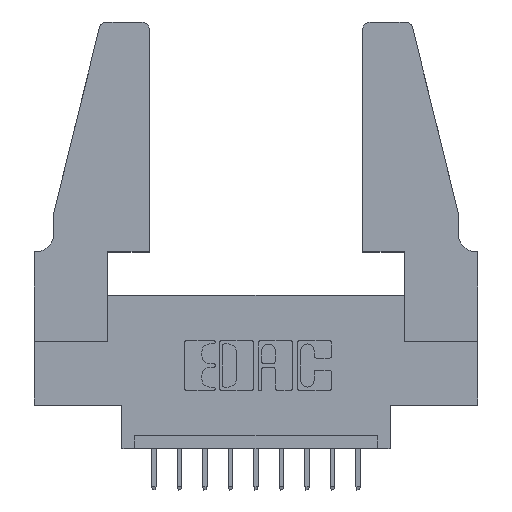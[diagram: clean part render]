
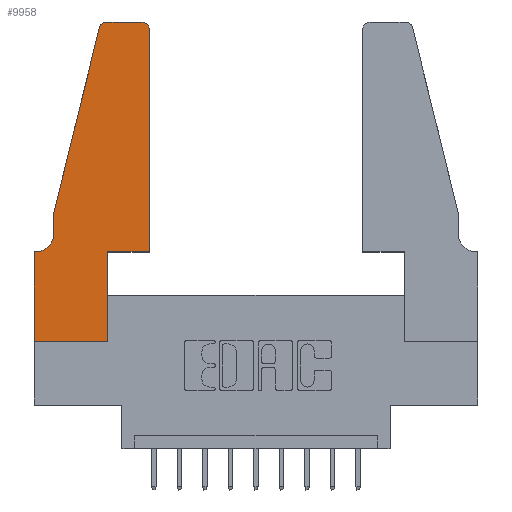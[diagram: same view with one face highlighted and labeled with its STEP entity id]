
A CAD part, top view. The second image highlights one B-rep face of the part: STEP entity #9958.
In plain terms, the highlighted planar face has unit normal (0, 0, 1).
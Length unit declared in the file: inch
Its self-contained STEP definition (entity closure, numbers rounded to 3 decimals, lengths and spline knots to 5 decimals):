
#3 = ORIENTED_EDGE ( 'NONE', *, *, #6358, .T. ) ;
#134 = CARTESIAN_POINT ( 'NONE',  ( 0.0755, 0.35, 0.37 ) ) ;
#165 = LINE ( 'NONE', #5622, #8355 ) ;
#537 = VERTEX_POINT ( 'NONE', #12414 ) ;
#626 = CARTESIAN_POINT ( 'NONE',  ( 0.0055, 0.42, 0.37 ) ) ;
#753 = CARTESIAN_POINT ( 'NONE',  ( 0.2865, 0.35, 0.37 ) ) ;
#811 = AXIS2_PLACEMENT_3D ( 'NONE', #626, #10054, #12198 ) ;
#1028 = VECTOR ( 'NONE', #9189, 39.37008 ) ;
#1066 = VERTEX_POINT ( 'NONE', #12648 ) ;
#1091 = EDGE_CURVE ( 'NONE', #8395, #537, #12053, .T. ) ;
#1284 = DIRECTION ( 'NONE',  ( -1., 0., 0. ) ) ;
#1615 = PLANE ( 'NONE',  #2673 ) ;
#1706 = VECTOR ( 'NONE', #11256, 39.37008 ) ;
#1890 = CARTESIAN_POINT ( 'NONE',  ( 0.4205, 1.22, 0.37 ) ) ;
#1960 = AXIS2_PLACEMENT_3D ( 'NONE', #6179, #8292, #2057 ) ;
#2007 = CARTESIAN_POINT ( 'NONE',  ( 0.0755, 0.5, 0.37 ) ) ;
#2057 = DIRECTION ( 'NONE',  ( 1., 0., 0. ) ) ;
#2092 = DIRECTION ( 'NONE',  ( 0., -1., 0. ) ) ;
#2666 = LINE ( 'NONE', #3909, #1706 ) ;
#2673 = AXIS2_PLACEMENT_3D ( 'NONE', #12162, #6963, #7012 ) ;
#2701 = CARTESIAN_POINT ( 'NONE',  ( 0.0055, 0.35, 0.37 ) ) ;
#2912 = EDGE_CURVE ( 'NONE', #3081, #7390, #2666, .T. ) ;
#2935 = VECTOR ( 'NONE', #3032, 39.37008 ) ;
#3032 = DIRECTION ( 'NONE',  ( -0.239, -0.971, 0. ) ) ;
#3081 = VERTEX_POINT ( 'NONE', #5078 ) ;
#3473 = EDGE_LOOP ( 'NONE', ( #4792, #3, #10211, #10979, #12687, #3763, #9276, #7944, #8809, #11815, #11348, #8243 ) ) ;
#3649 = VECTOR ( 'NONE', #7647, 39.37008 ) ;
#3763 = ORIENTED_EDGE ( 'NONE', *, *, #1091, .T. ) ;
#3909 = CARTESIAN_POINT ( 'NONE',  ( 0.4505, 0.35, 0.37 ) ) ;
#3953 = VERTEX_POINT ( 'NONE', #7107 ) ;
#4415 = EDGE_CURVE ( 'NONE', #11254, #12184, #8175, .T. ) ;
#4655 = LINE ( 'NONE', #12773, #3649 ) ;
#4792 = ORIENTED_EDGE ( 'NONE', *, *, #5617, .T. ) ;
#4809 = LINE ( 'NONE', #7193, #1028 ) ;
#5078 = CARTESIAN_POINT ( 'NONE',  ( 0.4505, 0.35, 0.37 ) ) ;
#5243 = EDGE_CURVE ( 'NONE', #1066, #8395, #11776, .T. ) ;
#5251 = DIRECTION ( 'NONE',  ( 1., 0., 0. ) ) ;
#5358 = EDGE_CURVE ( 'NONE', #3953, #8070, #4655, .T. ) ;
#5617 = EDGE_CURVE ( 'NONE', #11828, #8085, #165, .T. ) ;
#5622 = CARTESIAN_POINT ( 'NONE',  ( 0.2605, 1.25, 0.37 ) ) ;
#5999 = FACE_OUTER_BOUND ( 'NONE', #3473, .T. ) ;
#6179 = CARTESIAN_POINT ( 'NONE',  ( 0.284, 1.22, 0.37 ) ) ;
#6183 = VERTEX_POINT ( 'NONE', #10954 ) ;
#6358 = EDGE_CURVE ( 'NONE', #8085, #11254, #6907, .T. ) ;
#6853 = CARTESIAN_POINT ( 'NONE',  ( 0.4505, 1.22, 0.37 ) ) ;
#6907 = CIRCLE ( 'NONE', #1960, 0.03 ) ;
#6925 = CARTESIAN_POINT ( 'NONE',  ( 0.25487, 1.22718, 0.37 ) ) ;
#6963 = DIRECTION ( 'NONE',  ( 0., 0., 1. ) ) ;
#7012 = DIRECTION ( 'NONE',  ( 1., 0., 0. ) ) ;
#7107 = CARTESIAN_POINT ( 'NONE',  ( 0.2865, 0., 0.37 ) ) ;
#7193 = CARTESIAN_POINT ( 'NONE',  ( 0., 0., 0.37 ) ) ;
#7390 = VERTEX_POINT ( 'NONE', #6853 ) ;
#7647 = DIRECTION ( 'NONE',  ( 0., 1., 0. ) ) ;
#7944 = ORIENTED_EDGE ( 'NONE', *, *, #11393, .T. ) ;
#8070 = VERTEX_POINT ( 'NONE', #753 ) ;
#8085 = VERTEX_POINT ( 'NONE', #13191 ) ;
#8175 = LINE ( 'NONE', #9170, #2935 ) ;
#8232 = CARTESIAN_POINT ( 'NONE',  ( 0.4505, 0.35, 0.37 ) ) ;
#8243 = ORIENTED_EDGE ( 'NONE', *, *, #11944, .T. ) ;
#8292 = DIRECTION ( 'NONE',  ( 0., 0., 1. ) ) ;
#8355 = VECTOR ( 'NONE', #10848, 39.37008 ) ;
#8395 = VERTEX_POINT ( 'NONE', #2701 ) ;
#8534 = CARTESIAN_POINT ( 'NONE',  ( 0.4205, 1.25, 0.37 ) ) ;
#8809 = ORIENTED_EDGE ( 'NONE', *, *, #5358, .T. ) ;
#9170 = CARTESIAN_POINT ( 'NONE',  ( 0.0755, 0.5, 0.37 ) ) ;
#9189 = DIRECTION ( 'NONE',  ( 1., 0., 0. ) ) ;
#9276 = ORIENTED_EDGE ( 'NONE', *, *, #10500, .T. ) ;
#9361 = DIRECTION ( 'NONE',  ( 0., 0., 1. ) ) ;
#9629 = CARTESIAN_POINT ( 'NONE',  ( 0.0755, 0.5, 0.37 ) ) ;
#9958 = ADVANCED_FACE ( 'NONE', ( #5999 ), #1615, .T. ) ;
#10033 = LINE ( 'NONE', #2007, #12153 ) ;
#10054 = DIRECTION ( 'NONE',  ( 0., 0., -1. ) ) ;
#10211 = ORIENTED_EDGE ( 'NONE', *, *, #4415, .T. ) ;
#10332 = CARTESIAN_POINT ( 'NONE',  ( 0., 0., 0.37 ) ) ;
#10500 = EDGE_CURVE ( 'NONE', #537, #6183, #10542, .T. ) ;
#10542 = LINE ( 'NONE', #10332, #12498 ) ;
#10577 = EDGE_CURVE ( 'NONE', #8070, #3081, #12177, .T. ) ;
#10848 = DIRECTION ( 'NONE',  ( -1., 0., 0. ) ) ;
#10862 = AXIS2_PLACEMENT_3D ( 'NONE', #1890, #9361, #5251 ) ;
#10954 = CARTESIAN_POINT ( 'NONE',  ( 0., 0., 0.37 ) ) ;
#10979 = ORIENTED_EDGE ( 'NONE', *, *, #11449, .T. ) ;
#11254 = VERTEX_POINT ( 'NONE', #6925 ) ;
#11256 = DIRECTION ( 'NONE',  ( 0., 1., 0. ) ) ;
#11348 = ORIENTED_EDGE ( 'NONE', *, *, #2912, .T. ) ;
#11393 = EDGE_CURVE ( 'NONE', #6183, #3953, #4809, .T. ) ;
#11449 = EDGE_CURVE ( 'NONE', #12184, #1066, #10033, .T. ) ;
#11776 = CIRCLE ( 'NONE', #811, 0.07 ) ;
#11815 = ORIENTED_EDGE ( 'NONE', *, *, #10577, .T. ) ;
#11828 = VERTEX_POINT ( 'NONE', #8534 ) ;
#11885 = VECTOR ( 'NONE', #1284, 39.37008 ) ;
#11944 = EDGE_CURVE ( 'NONE', #7390, #11828, #13021, .T. ) ;
#12053 = LINE ( 'NONE', #134, #11885 ) ;
#12153 = VECTOR ( 'NONE', #12324, 39.37008 ) ;
#12162 = CARTESIAN_POINT ( 'NONE',  ( 0., 0.35, 0.37 ) ) ;
#12177 = LINE ( 'NONE', #8232, #12346 ) ;
#12184 = VERTEX_POINT ( 'NONE', #9629 ) ;
#12198 = DIRECTION ( 'NONE',  ( -1., 0., 0. ) ) ;
#12324 = DIRECTION ( 'NONE',  ( 0., -1., 0. ) ) ;
#12346 = VECTOR ( 'NONE', #13329, 39.37008 ) ;
#12414 = CARTESIAN_POINT ( 'NONE',  ( 0., 0.35, 0.37 ) ) ;
#12498 = VECTOR ( 'NONE', #2092, 39.37008 ) ;
#12648 = CARTESIAN_POINT ( 'NONE',  ( 0.0755, 0.42, 0.37 ) ) ;
#12687 = ORIENTED_EDGE ( 'NONE', *, *, #5243, .T. ) ;
#12773 = CARTESIAN_POINT ( 'NONE',  ( 0.2865, 0.35, 0.37 ) ) ;
#13021 = CIRCLE ( 'NONE', #10862, 0.03 ) ;
#13191 = CARTESIAN_POINT ( 'NONE',  ( 0.284, 1.25, 0.37 ) ) ;
#13329 = DIRECTION ( 'NONE',  ( 1., 0., 0. ) ) ;
